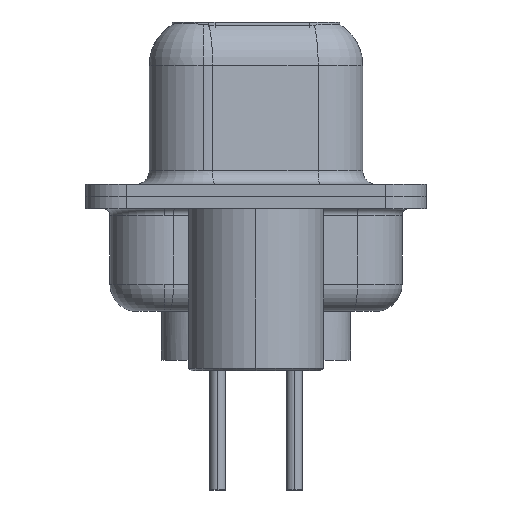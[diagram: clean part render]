
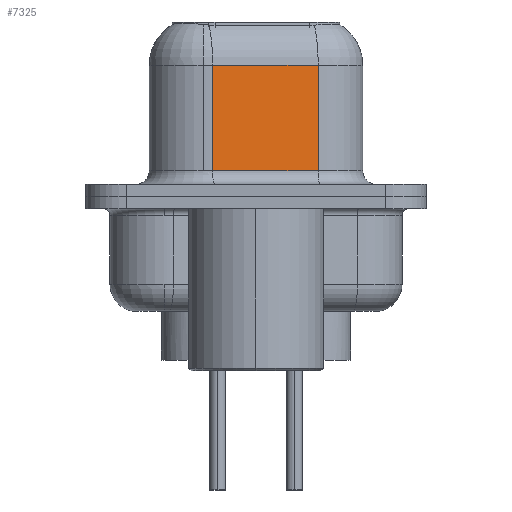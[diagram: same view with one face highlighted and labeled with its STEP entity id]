
A CAD part, left-side view. The second image highlights one B-rep face of the part: STEP entity #7325.
In plain terms, the highlighted planar face has unit normal (-0.985, -0.174, 0).
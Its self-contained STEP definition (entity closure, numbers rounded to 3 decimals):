
#938 = CARTESIAN_POINT ( 'NONE',  ( 5.063, -2.297, 0.95 ) ) ;
#1244 = ORIENTED_EDGE ( 'NONE', *, *, #14759, .T. ) ;
#2067 = VERTEX_POINT ( 'NONE', #18368 ) ;
#2845 = CARTESIAN_POINT ( 'NONE',  ( 5.063, -2.297, 0.95 ) ) ;
#3389 = VECTOR ( 'NONE', #10334, 1000. ) ;
#3469 = LINE ( 'NONE', #13615, #3389 ) ;
#3729 = VECTOR ( 'NONE', #4625, 1000. ) ;
#4399 = VERTEX_POINT ( 'NONE', #17188 ) ;
#4625 = DIRECTION ( 'NONE',  ( 0., 0., -1. ) ) ;
#4708 = DIRECTION ( 'NONE',  ( -0.174, 0.985, 0. ) ) ;
#5140 = EDGE_CURVE ( 'NONE', #2067, #10027, #3469, .T. ) ;
#6186 = FACE_OUTER_BOUND ( 'NONE', #9236, .T. ) ;
#6325 = LINE ( 'NONE', #10023, #3729 ) ;
#6945 = EDGE_CURVE ( 'NONE', #10367, #4399, #6325, .T. ) ;
#7325 = ADVANCED_FACE ( 'NONE', ( #6186 ), #19928, .F. ) ;
#7617 = DIRECTION ( 'NONE',  ( -0.174, 0.985, 0. ) ) ;
#7813 = DIRECTION ( 'NONE',  ( 0.174, -0.985, 0. ) ) ;
#8263 = ORIENTED_EDGE ( 'NONE', *, *, #21638, .T. ) ;
#8575 = ORIENTED_EDGE ( 'NONE', *, *, #6945, .T. ) ;
#9236 = EDGE_LOOP ( 'NONE', ( #18442, #8263, #8575, #1244 ) ) ;
#10023 = CARTESIAN_POINT ( 'NONE',  ( 4.375, 1.603, 6.6 ) ) ;
#10027 = VERTEX_POINT ( 'NONE', #2845 ) ;
#10334 = DIRECTION ( 'NONE',  ( 0., 0., -1. ) ) ;
#10367 = VERTEX_POINT ( 'NONE', #12384 ) ;
#10748 = CARTESIAN_POINT ( 'NONE',  ( 5.063, -2.297, 4.85 ) ) ;
#12384 = CARTESIAN_POINT ( 'NONE',  ( 4.375, 1.603, 4.85 ) ) ;
#13128 = AXIS2_PLACEMENT_3D ( 'NONE', #13276, #16875, #4708 ) ;
#13214 = LINE ( 'NONE', #938, #13645 ) ;
#13276 = CARTESIAN_POINT ( 'NONE',  ( 5.063, -2.297, 6.6 ) ) ;
#13615 = CARTESIAN_POINT ( 'NONE',  ( 5.063, -2.297, 6.6 ) ) ;
#13645 = VECTOR ( 'NONE', #7813, 1000. ) ;
#14759 = EDGE_CURVE ( 'NONE', #4399, #10027, #13214, .T. ) ;
#16875 = DIRECTION ( 'NONE',  ( 0.985, 0.174, 0. ) ) ;
#17188 = CARTESIAN_POINT ( 'NONE',  ( 4.375, 1.603, 0.95 ) ) ;
#17368 = VECTOR ( 'NONE', #7617, 1000. ) ;
#18368 = CARTESIAN_POINT ( 'NONE',  ( 5.063, -2.297, 4.85 ) ) ;
#18442 = ORIENTED_EDGE ( 'NONE', *, *, #5140, .F. ) ;
#19928 = PLANE ( 'NONE',  #13128 ) ;
#21019 = LINE ( 'NONE', #10748, #17368 ) ;
#21638 = EDGE_CURVE ( 'NONE', #2067, #10367, #21019, .T. ) ;
